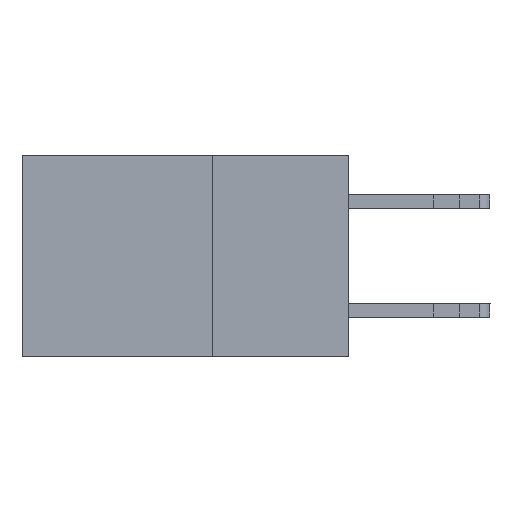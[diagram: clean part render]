
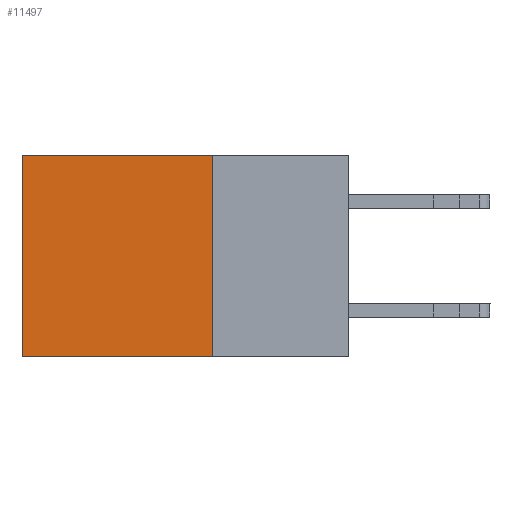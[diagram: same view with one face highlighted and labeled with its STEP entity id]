
A CAD part, left-side view. The second image highlights one B-rep face of the part: STEP entity #11497.
In plain terms, the highlighted planar face has unit normal (-1, 0, 0).
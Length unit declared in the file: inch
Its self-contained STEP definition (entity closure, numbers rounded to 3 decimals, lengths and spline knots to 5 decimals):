
#1347 = DIRECTION ( 'NONE',  ( 0., 1., 0. ) ) ;
#2339 = CARTESIAN_POINT ( 'NONE',  ( 0.298, 0.25, -0.37 ) ) ;
#2394 = VECTOR ( 'NONE', #5005, 39.37008 ) ;
#2808 = CARTESIAN_POINT ( 'NONE',  ( 0.298, 0.6, 0. ) ) ;
#2829 = VERTEX_POINT ( 'NONE', #15623 ) ;
#3236 = EDGE_CURVE ( 'NONE', #2829, #12138, #16137, .T. ) ;
#3789 = VECTOR ( 'NONE', #10810, 39.37008 ) ;
#4327 = AXIS2_PLACEMENT_3D ( 'NONE', #5241, #18739, #12772 ) ;
#4730 = EDGE_CURVE ( 'NONE', #16867, #14209, #9731, .T. ) ;
#4784 = CARTESIAN_POINT ( 'NONE',  ( 0.298, 0.25, -0.37 ) ) ;
#5005 = DIRECTION ( 'NONE',  ( 0., 0., -1. ) ) ;
#5241 = CARTESIAN_POINT ( 'NONE',  ( 0.298, 0.25, 0. ) ) ;
#5715 = LINE ( 'NONE', #14076, #2394 ) ;
#6397 = LINE ( 'NONE', #11455, #17311 ) ;
#6806 = DIRECTION ( 'NONE',  ( 0., 0., -1. ) ) ;
#6900 = ORIENTED_EDGE ( 'NONE', *, *, #8144, .T. ) ;
#8144 = EDGE_CURVE ( 'NONE', #12138, #14209, #6397, .T. ) ;
#8172 = PLANE ( 'NONE',  #4327 ) ;
#9043 = VECTOR ( 'NONE', #1347, 39.37008 ) ;
#9731 = LINE ( 'NONE', #4784, #3789 ) ;
#10810 = DIRECTION ( 'NONE',  ( 0., 1., 0. ) ) ;
#11168 = ORIENTED_EDGE ( 'NONE', *, *, #4730, .F. ) ;
#11455 = CARTESIAN_POINT ( 'NONE',  ( 0.298, 0.6, 0. ) ) ;
#11497 = ADVANCED_FACE ( 'NONE', ( #14764 ), #8172, .F. ) ;
#11938 = ORIENTED_EDGE ( 'NONE', *, *, #13206, .F. ) ;
#12138 = VERTEX_POINT ( 'NONE', #2808 ) ;
#12772 = DIRECTION ( 'NONE',  ( 0., 0., -1. ) ) ;
#13206 = EDGE_CURVE ( 'NONE', #2829, #16867, #5715, .T. ) ;
#13420 = CARTESIAN_POINT ( 'NONE',  ( 0.298, 0.25, 0. ) ) ;
#14076 = CARTESIAN_POINT ( 'NONE',  ( 0.298, 0.25, 0. ) ) ;
#14081 = ORIENTED_EDGE ( 'NONE', *, *, #3236, .T. ) ;
#14209 = VERTEX_POINT ( 'NONE', #15013 ) ;
#14764 = FACE_OUTER_BOUND ( 'NONE', #15975, .T. ) ;
#15013 = CARTESIAN_POINT ( 'NONE',  ( 0.298, 0.6, -0.37 ) ) ;
#15623 = CARTESIAN_POINT ( 'NONE',  ( 0.298, 0.25, 0. ) ) ;
#15975 = EDGE_LOOP ( 'NONE', ( #6900, #11168, #11938, #14081 ) ) ;
#16137 = LINE ( 'NONE', #13420, #9043 ) ;
#16867 = VERTEX_POINT ( 'NONE', #2339 ) ;
#17311 = VECTOR ( 'NONE', #6806, 39.37008 ) ;
#18739 = DIRECTION ( 'NONE',  ( 1., 0., 0. ) ) ;
